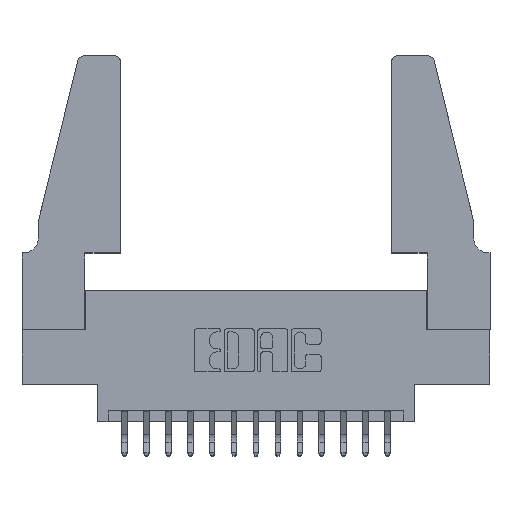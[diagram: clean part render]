
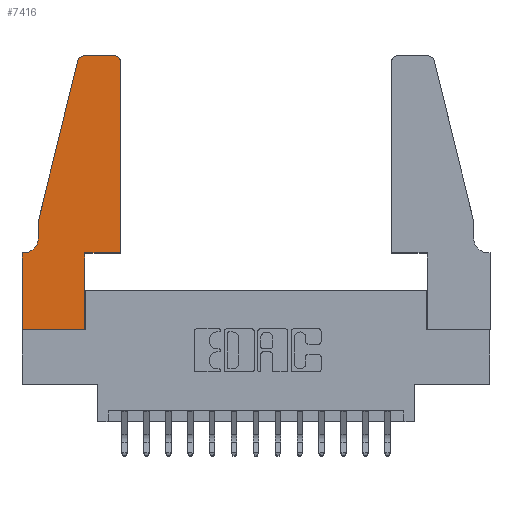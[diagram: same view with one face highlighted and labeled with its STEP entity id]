
A CAD part, top view. The second image highlights one B-rep face of the part: STEP entity #7416.
In plain terms, the highlighted planar face has unit normal (0, 0, 1).
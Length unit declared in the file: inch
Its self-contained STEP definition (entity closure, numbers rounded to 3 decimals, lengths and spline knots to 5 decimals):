
#81 = CARTESIAN_POINT ( 'NONE',  ( 0.284, 1.22, 0.37 ) ) ;
#85 = VERTEX_POINT ( 'NONE', #5919 ) ;
#238 = ORIENTED_EDGE ( 'NONE', *, *, #6867, .T. ) ;
#444 = CARTESIAN_POINT ( 'NONE',  ( 0.0755, 0.5, 0.37 ) ) ;
#483 = CARTESIAN_POINT ( 'NONE',  ( 0.2865, 0.35, 0.37 ) ) ;
#578 = CARTESIAN_POINT ( 'NONE',  ( 0.4505, 1.22, 0.37 ) ) ;
#649 = LINE ( 'NONE', #6658, #2459 ) ;
#1183 = CARTESIAN_POINT ( 'NONE',  ( 0.4505, 0.35, 0.37 ) ) ;
#1194 = VERTEX_POINT ( 'NONE', #15698 ) ;
#1339 = EDGE_CURVE ( 'NONE', #16047, #5499, #4066, .T. ) ;
#1510 = LINE ( 'NONE', #2653, #14366 ) ;
#1577 = DIRECTION ( 'NONE',  ( 0., -1., 0. ) ) ;
#1795 = VERTEX_POINT ( 'NONE', #9844 ) ;
#2076 = DIRECTION ( 'NONE',  ( 1., 0., 0. ) ) ;
#2439 = EDGE_CURVE ( 'NONE', #12857, #85, #15878, .T. ) ;
#2459 = VECTOR ( 'NONE', #6809, 39.37008 ) ;
#2508 = ORIENTED_EDGE ( 'NONE', *, *, #1339, .T. ) ;
#2514 = VERTEX_POINT ( 'NONE', #6810 ) ;
#2653 = CARTESIAN_POINT ( 'NONE',  ( 0.4505, 0.35, 0.37 ) ) ;
#2830 = DIRECTION ( 'NONE',  ( 0., 0., 1. ) ) ;
#2897 = AXIS2_PLACEMENT_3D ( 'NONE', #81, #2830, #5286 ) ;
#2965 = EDGE_CURVE ( 'NONE', #1795, #14437, #11669, .T. ) ;
#3104 = DIRECTION ( 'NONE',  ( 1., 0., 0. ) ) ;
#3307 = DIRECTION ( 'NONE',  ( 0., 0., 1. ) ) ;
#3600 = CARTESIAN_POINT ( 'NONE',  ( 0., 0.35, 0.37 ) ) ;
#4066 = LINE ( 'NONE', #5665, #11712 ) ;
#4193 = LINE ( 'NONE', #444, #16449 ) ;
#4236 = AXIS2_PLACEMENT_3D ( 'NONE', #3600, #7468, #16181 ) ;
#4445 = VECTOR ( 'NONE', #16276, 39.37008 ) ;
#4478 = CIRCLE ( 'NONE', #14344, 0.07 ) ;
#4515 = CARTESIAN_POINT ( 'NONE',  ( 0.0755, 0.42, 0.37 ) ) ;
#4739 = ORIENTED_EDGE ( 'NONE', *, *, #15417, .T. ) ;
#5051 = LINE ( 'NONE', #11163, #10273 ) ;
#5266 = CARTESIAN_POINT ( 'NONE',  ( 0.0055, 0.42, 0.37 ) ) ;
#5286 = DIRECTION ( 'NONE',  ( 1., 0., 0. ) ) ;
#5499 = VERTEX_POINT ( 'NONE', #1183 ) ;
#5578 = VERTEX_POINT ( 'NONE', #10036 ) ;
#5641 = AXIS2_PLACEMENT_3D ( 'NONE', #7290, #3307, #2076 ) ;
#5665 = CARTESIAN_POINT ( 'NONE',  ( 0.4505, 0.35, 0.37 ) ) ;
#5675 = ORIENTED_EDGE ( 'NONE', *, *, #11392, .T. ) ;
#5865 = DIRECTION ( 'NONE',  ( -1., 0., 0. ) ) ;
#5919 = CARTESIAN_POINT ( 'NONE',  ( 0.284, 1.25, 0.37 ) ) ;
#6033 = LINE ( 'NONE', #9332, #12824 ) ;
#6101 = EDGE_CURVE ( 'NONE', #5578, #11607, #13328, .T. ) ;
#6282 = VECTOR ( 'NONE', #5865, 39.37008 ) ;
#6436 = VERTEX_POINT ( 'NONE', #578 ) ;
#6576 = DIRECTION ( 'NONE',  ( 0., 1., 0. ) ) ;
#6605 = ORIENTED_EDGE ( 'NONE', *, *, #2439, .T. ) ;
#6658 = CARTESIAN_POINT ( 'NONE',  ( 0., 0., 0.37 ) ) ;
#6809 = DIRECTION ( 'NONE',  ( 1., 0., 0. ) ) ;
#6810 = CARTESIAN_POINT ( 'NONE',  ( 0.2865, 0., 0.37 ) ) ;
#6867 = EDGE_CURVE ( 'NONE', #1194, #2514, #649, .T. ) ;
#6972 = EDGE_CURVE ( 'NONE', #11607, #1795, #4478, .T. ) ;
#7089 = CARTESIAN_POINT ( 'NONE',  ( 0.4205, 1.25, 0.37 ) ) ;
#7290 = CARTESIAN_POINT ( 'NONE',  ( 0.4205, 1.22, 0.37 ) ) ;
#7364 = PLANE ( 'NONE',  #4236 ) ;
#7416 = ADVANCED_FACE ( 'NONE', ( #10687 ), #7364, .T. ) ;
#7468 = DIRECTION ( 'NONE',  ( 0., 0., 1. ) ) ;
#7624 = ORIENTED_EDGE ( 'NONE', *, *, #2965, .T. ) ;
#7668 = CIRCLE ( 'NONE', #2897, 0.03 ) ;
#7831 = ORIENTED_EDGE ( 'NONE', *, *, #6101, .T. ) ;
#9105 = EDGE_CURVE ( 'NONE', #2514, #16047, #5051, .T. ) ;
#9332 = CARTESIAN_POINT ( 'NONE',  ( 0., 0., 0.37 ) ) ;
#9447 = DIRECTION ( 'NONE',  ( 0., -1., 0. ) ) ;
#9844 = CARTESIAN_POINT ( 'NONE',  ( 0.0055, 0.35, 0.37 ) ) ;
#9904 = ORIENTED_EDGE ( 'NONE', *, *, #9105, .T. ) ;
#9987 = EDGE_CURVE ( 'NONE', #14437, #1194, #6033, .T. ) ;
#10036 = CARTESIAN_POINT ( 'NONE',  ( 0.0755, 0.5, 0.37 ) ) ;
#10234 = ORIENTED_EDGE ( 'NONE', *, *, #6972, .T. ) ;
#10273 = VECTOR ( 'NONE', #6576, 39.37008 ) ;
#10415 = CARTESIAN_POINT ( 'NONE',  ( 0.0755, 0.5, 0.37 ) ) ;
#10687 = FACE_OUTER_BOUND ( 'NONE', #15619, .T. ) ;
#10977 = DIRECTION ( 'NONE',  ( -0.239, -0.971, 0. ) ) ;
#10987 = ORIENTED_EDGE ( 'NONE', *, *, #15478, .T. ) ;
#11163 = CARTESIAN_POINT ( 'NONE',  ( 0.2865, 0.35, 0.37 ) ) ;
#11239 = CARTESIAN_POINT ( 'NONE',  ( 0.2605, 1.25, 0.37 ) ) ;
#11392 = EDGE_CURVE ( 'NONE', #5499, #6436, #1510, .T. ) ;
#11607 = VERTEX_POINT ( 'NONE', #4515 ) ;
#11669 = LINE ( 'NONE', #14995, #4445 ) ;
#11712 = VECTOR ( 'NONE', #3104, 39.37008 ) ;
#11745 = DIRECTION ( 'NONE',  ( 0., 0., -1. ) ) ;
#12039 = CARTESIAN_POINT ( 'NONE',  ( 0.25487, 1.22718, 0.37 ) ) ;
#12733 = VECTOR ( 'NONE', #1577, 39.37008 ) ;
#12824 = VECTOR ( 'NONE', #9447, 39.37008 ) ;
#12857 = VERTEX_POINT ( 'NONE', #7089 ) ;
#13328 = LINE ( 'NONE', #10415, #12733 ) ;
#13449 = CIRCLE ( 'NONE', #5641, 0.03 ) ;
#14203 = DIRECTION ( 'NONE',  ( -1., 0., 0. ) ) ;
#14285 = CARTESIAN_POINT ( 'NONE',  ( 0., 0.35, 0.37 ) ) ;
#14344 = AXIS2_PLACEMENT_3D ( 'NONE', #5266, #11745, #14203 ) ;
#14349 = ORIENTED_EDGE ( 'NONE', *, *, #9987, .T. ) ;
#14366 = VECTOR ( 'NONE', #15450, 39.37008 ) ;
#14437 = VERTEX_POINT ( 'NONE', #14285 ) ;
#14507 = EDGE_CURVE ( 'NONE', #85, #14636, #7668, .T. ) ;
#14636 = VERTEX_POINT ( 'NONE', #12039 ) ;
#14995 = CARTESIAN_POINT ( 'NONE',  ( 0.0755, 0.35, 0.37 ) ) ;
#15417 = EDGE_CURVE ( 'NONE', #14636, #5578, #4193, .T. ) ;
#15450 = DIRECTION ( 'NONE',  ( 0., 1., 0. ) ) ;
#15478 = EDGE_CURVE ( 'NONE', #6436, #12857, #13449, .T. ) ;
#15619 = EDGE_LOOP ( 'NONE', ( #6605, #16473, #4739, #7831, #10234, #7624, #14349, #238, #9904, #2508, #5675, #10987 ) ) ;
#15698 = CARTESIAN_POINT ( 'NONE',  ( 0., 0., 0.37 ) ) ;
#15878 = LINE ( 'NONE', #11239, #6282 ) ;
#16047 = VERTEX_POINT ( 'NONE', #483 ) ;
#16181 = DIRECTION ( 'NONE',  ( 1., 0., 0. ) ) ;
#16276 = DIRECTION ( 'NONE',  ( -1., 0., 0. ) ) ;
#16449 = VECTOR ( 'NONE', #10977, 39.37008 ) ;
#16473 = ORIENTED_EDGE ( 'NONE', *, *, #14507, .T. ) ;
